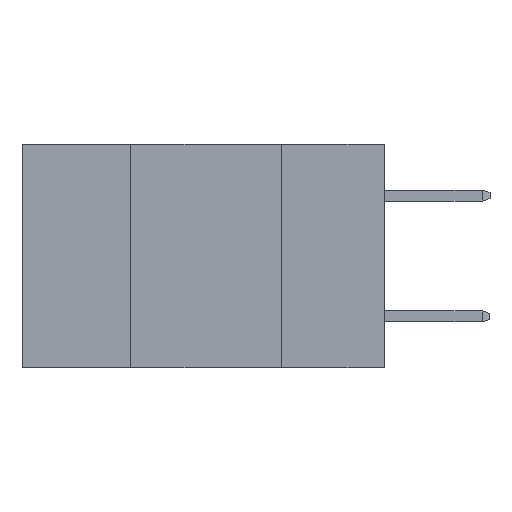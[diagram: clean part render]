
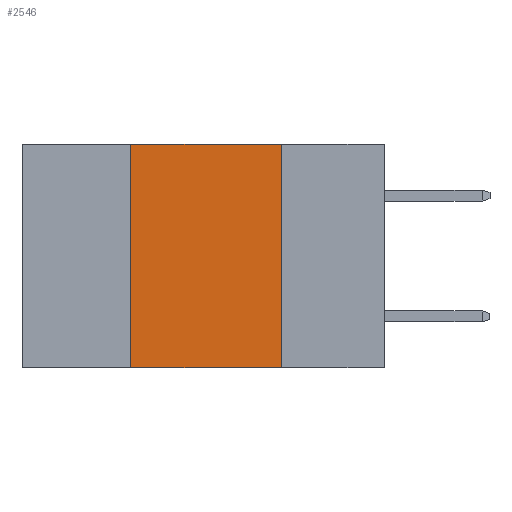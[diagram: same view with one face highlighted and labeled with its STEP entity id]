
A CAD part, left-side view. The second image highlights one B-rep face of the part: STEP entity #2546.
In plain terms, the highlighted planar face has unit normal (-1, 0, 0).
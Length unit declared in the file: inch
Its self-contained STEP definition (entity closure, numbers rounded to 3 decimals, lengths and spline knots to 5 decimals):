
#1690 = VECTOR ( 'NONE', #12428, 39.37008 ) ;
#1858 = CARTESIAN_POINT ( 'NONE',  ( 0., 0.42, -0.37 ) ) ;
#1989 = EDGE_CURVE ( 'NONE', #6544, #6576, #11824, .T. ) ;
#2190 = CARTESIAN_POINT ( 'NONE',  ( 0., 0.6, -0.37 ) ) ;
#2546 = ADVANCED_FACE ( 'NONE', ( #13182 ), #11410, .F. ) ;
#2739 = CARTESIAN_POINT ( 'NONE',  ( 0., 0.17, 0. ) ) ;
#2982 = VERTEX_POINT ( 'NONE', #1858 ) ;
#3200 = DIRECTION ( 'NONE',  ( 0., 0., -1. ) ) ;
#3538 = VECTOR ( 'NONE', #10073, 39.37008 ) ;
#3833 = CARTESIAN_POINT ( 'NONE',  ( 0., 0.42, 0. ) ) ;
#4418 = EDGE_CURVE ( 'NONE', #2982, #6544, #5428, .T. ) ;
#4517 = DIRECTION ( 'NONE',  ( 0., -1., 0. ) ) ;
#5227 = VERTEX_POINT ( 'NONE', #10006 ) ;
#5428 = LINE ( 'NONE', #9852, #13135 ) ;
#6343 = LINE ( 'NONE', #2739, #3538 ) ;
#6544 = VERTEX_POINT ( 'NONE', #3833 ) ;
#6576 = VERTEX_POINT ( 'NONE', #10026 ) ;
#6706 = DIRECTION ( 'NONE',  ( 0., 0., 1. ) ) ;
#7106 = ORIENTED_EDGE ( 'NONE', *, *, #12978, .F. ) ;
#7581 = CARTESIAN_POINT ( 'NONE',  ( 0., 0.6, 0. ) ) ;
#7767 = ORIENTED_EDGE ( 'NONE', *, *, #12081, .T. ) ;
#8893 = VECTOR ( 'NONE', #4517, 39.37008 ) ;
#9837 = ORIENTED_EDGE ( 'NONE', *, *, #1989, .F. ) ;
#9852 = CARTESIAN_POINT ( 'NONE',  ( 0., 0.42, 0. ) ) ;
#10006 = CARTESIAN_POINT ( 'NONE',  ( 0., 0.17, -0.37 ) ) ;
#10026 = CARTESIAN_POINT ( 'NONE',  ( 0., 0.17, 0. ) ) ;
#10073 = DIRECTION ( 'NONE',  ( 0., 0., -1. ) ) ;
#10211 = DIRECTION ( 'NONE',  ( 1., 0., 0. ) ) ;
#11335 = EDGE_LOOP ( 'NONE', ( #7106, #9837, #12740, #7767 ) ) ;
#11410 = PLANE ( 'NONE',  #12303 ) ;
#11657 = CARTESIAN_POINT ( 'NONE',  ( 0., 0.6, 0. ) ) ;
#11824 = LINE ( 'NONE', #11657, #8893 ) ;
#12081 = EDGE_CURVE ( 'NONE', #2982, #5227, #12329, .T. ) ;
#12303 = AXIS2_PLACEMENT_3D ( 'NONE', #7581, #10211, #3200 ) ;
#12329 = LINE ( 'NONE', #2190, #1690 ) ;
#12428 = DIRECTION ( 'NONE',  ( 0., -1., 0. ) ) ;
#12740 = ORIENTED_EDGE ( 'NONE', *, *, #4418, .F. ) ;
#12978 = EDGE_CURVE ( 'NONE', #6576, #5227, #6343, .T. ) ;
#13135 = VECTOR ( 'NONE', #6706, 39.37008 ) ;
#13182 = FACE_OUTER_BOUND ( 'NONE', #11335, .T. ) ;
